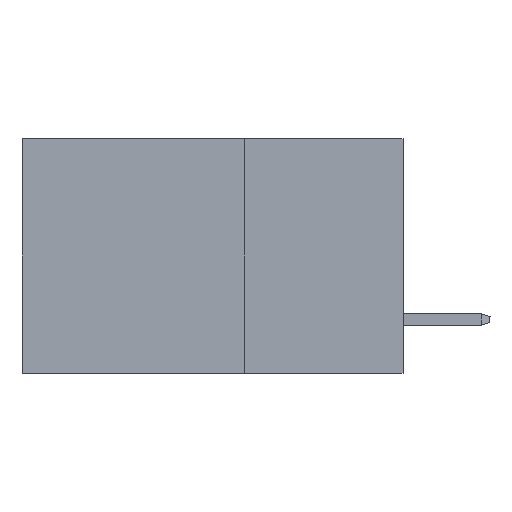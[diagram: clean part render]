
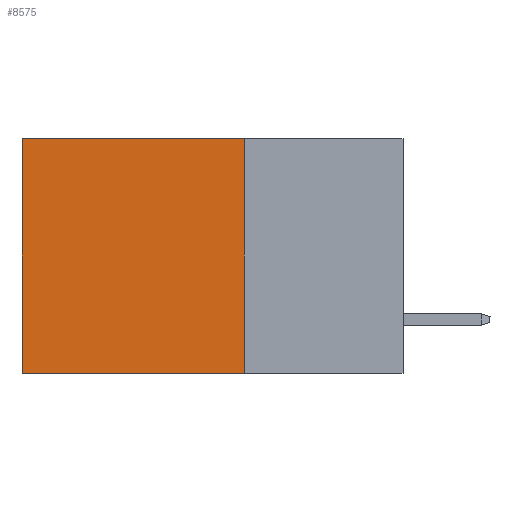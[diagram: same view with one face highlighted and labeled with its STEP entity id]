
A CAD part, left-side view. The second image highlights one B-rep face of the part: STEP entity #8575.
In plain terms, the highlighted planar face has unit normal (-1, 0, 0).
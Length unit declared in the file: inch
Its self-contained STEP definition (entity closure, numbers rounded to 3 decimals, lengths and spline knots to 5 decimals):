
#713 = VECTOR ( 'NONE', #2363, 39.37008 ) ;
#2081 = ORIENTED_EDGE ( 'NONE', *, *, #5849, .F. ) ;
#2363 = DIRECTION ( 'NONE',  ( 0., 0., -1. ) ) ;
#2554 = DIRECTION ( 'NONE',  ( 0., 1., 0. ) ) ;
#2760 = ORIENTED_EDGE ( 'NONE', *, *, #6139, .T. ) ;
#2982 = LINE ( 'NONE', #25701, #24345 ) ;
#5035 = ORIENTED_EDGE ( 'NONE', *, *, #10219, .T. ) ;
#5395 = DIRECTION ( 'NONE',  ( 0., 0., -1. ) ) ;
#5787 = VECTOR ( 'NONE', #2554, 39.37008 ) ;
#5849 = EDGE_CURVE ( 'NONE', #6392, #8481, #2982, .T. ) ;
#5896 = CARTESIAN_POINT ( 'NONE',  ( 0.2875, 0.25, -0.37 ) ) ;
#6139 = EDGE_CURVE ( 'NONE', #6392, #16426, #8751, .T. ) ;
#6392 = VERTEX_POINT ( 'NONE', #18312 ) ;
#8457 = CARTESIAN_POINT ( 'NONE',  ( 0.2875, 0.25, 0. ) ) ;
#8481 = VERTEX_POINT ( 'NONE', #5896 ) ;
#8575 = ADVANCED_FACE ( 'NONE', ( #16829 ), #10344, .F. ) ;
#8751 = LINE ( 'NONE', #25129, #5787 ) ;
#9425 = CARTESIAN_POINT ( 'NONE',  ( 0.2875, 0.6, 0. ) ) ;
#10219 = EDGE_CURVE ( 'NONE', #16426, #17603, #19687, .T. ) ;
#10344 = PLANE ( 'NONE',  #18318 ) ;
#10619 = EDGE_LOOP ( 'NONE', ( #5035, #13643, #2081, #2760 ) ) ;
#12221 = CARTESIAN_POINT ( 'NONE',  ( 0.2875, 0.25, -0.37 ) ) ;
#12780 = DIRECTION ( 'NONE',  ( 0., 0., -1. ) ) ;
#13643 = ORIENTED_EDGE ( 'NONE', *, *, #26394, .F. ) ;
#16426 = VERTEX_POINT ( 'NONE', #23974 ) ;
#16829 = FACE_OUTER_BOUND ( 'NONE', #10619, .T. ) ;
#17216 = CARTESIAN_POINT ( 'NONE',  ( 0.2875, 0.6, -0.37 ) ) ;
#17603 = VERTEX_POINT ( 'NONE', #17216 ) ;
#18293 = LINE ( 'NONE', #12221, #24302 ) ;
#18312 = CARTESIAN_POINT ( 'NONE',  ( 0.2875, 0.25, 0. ) ) ;
#18318 = AXIS2_PLACEMENT_3D ( 'NONE', #8457, #22656, #12780 ) ;
#18562 = DIRECTION ( 'NONE',  ( 0., 1., 0. ) ) ;
#19687 = LINE ( 'NONE', #9425, #713 ) ;
#22656 = DIRECTION ( 'NONE',  ( 1., 0., 0. ) ) ;
#23974 = CARTESIAN_POINT ( 'NONE',  ( 0.2875, 0.6, 0. ) ) ;
#24302 = VECTOR ( 'NONE', #18562, 39.37008 ) ;
#24345 = VECTOR ( 'NONE', #5395, 39.37008 ) ;
#25129 = CARTESIAN_POINT ( 'NONE',  ( 0.2875, 0.25, 0. ) ) ;
#25701 = CARTESIAN_POINT ( 'NONE',  ( 0.2875, 0.25, 0. ) ) ;
#26394 = EDGE_CURVE ( 'NONE', #8481, #17603, #18293, .T. ) ;
